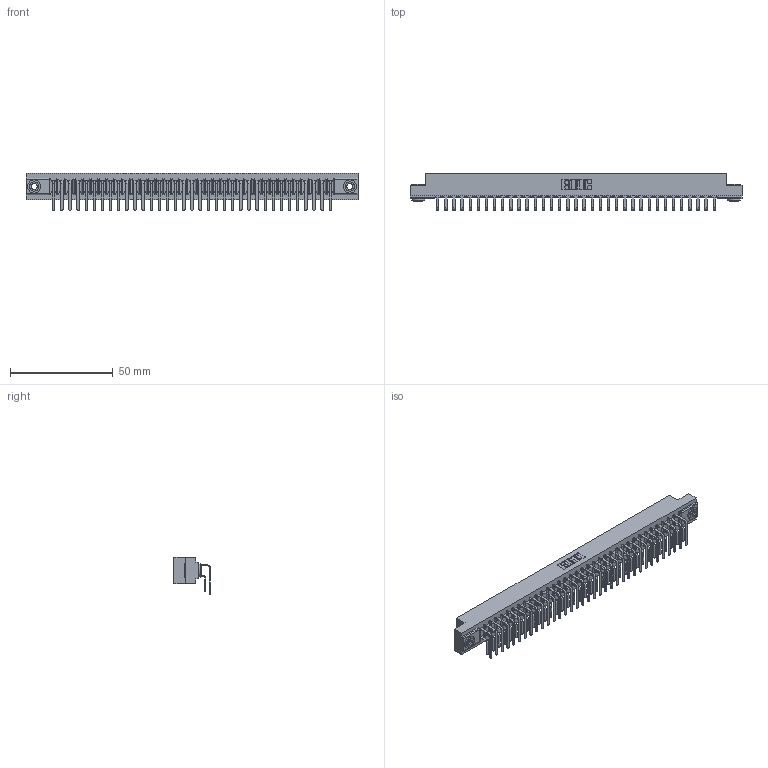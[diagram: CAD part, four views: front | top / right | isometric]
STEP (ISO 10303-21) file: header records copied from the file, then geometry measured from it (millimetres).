
FILE_DESCRIPTION (( 'STEP AP203' ), '1' );
FILE_NAME ('307-070-459-203.STEP', '2020-10-01T00:52:40', ( '' ), ( '' ), 'SwSTEP 2.0', 'SolidWorks 2020', '' );
FILE_SCHEMA (( 'CONFIG_CONTROL_DESIGN' ));
Length unit declared in the file: inch
Products named in the file (5): 307 Part_.156 Dia Mounting Holes; 307-070-459-203; 345-250-002_345-250-002-102; 307-290-001_558 559 - 1 (Single); 307-290-001_559 - 2 (Single)
Assembly tree (73 placements, depth 2):
  307-070-459-203
    307 Part_.156 Dia Mounting Holes
    307-290-001_558 559 - 1 (Single)  x35
    307-290-001_559 - 2 (Single)  x35
    345-250-002_345-250-002-102  x2
Bounding box: 161.7 x 17.69 x 18.07 mm (x, y, z)
Volume: 17456.5 mm3; surface area: 23276.1 mm2
Topology: 73 solids, 73 shells, 3706 faces, 10375 edges, 6722 vertices
Faces by surface type: plane 2404, cylinder 1222, sphere 72, cone 8
Entity records: 34500 total; most frequent: CARTESIAN_POINT 5630, ORIENTED_EDGE 5570, DIRECTION 5531, EDGE_CURVE 2785, VECTOR 2125, LINE 2125, VERTEX_POINT 1802, AXIS2_PLACEMENT_3D 1703
